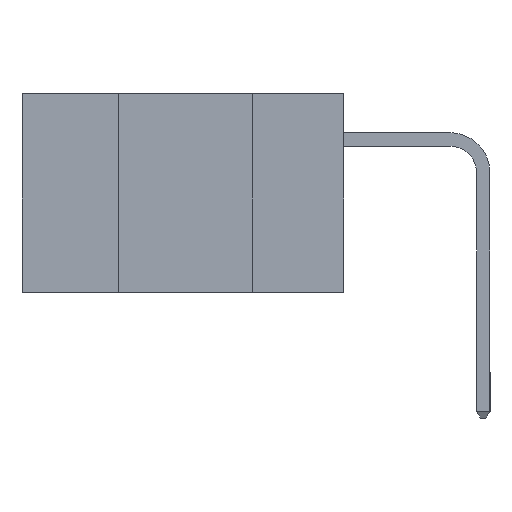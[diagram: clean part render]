
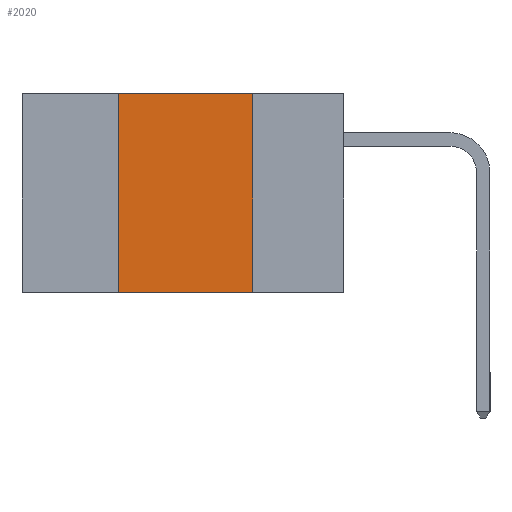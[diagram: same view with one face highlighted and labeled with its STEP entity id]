
A CAD part, left-side view. The second image highlights one B-rep face of the part: STEP entity #2020.
In plain terms, the highlighted planar face has unit normal (-1, 0, 0).
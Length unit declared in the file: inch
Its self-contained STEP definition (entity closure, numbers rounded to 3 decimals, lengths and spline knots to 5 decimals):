
#37 = CARTESIAN_POINT ( 'NONE',  ( 0., 0.6, 0. ) ) ;
#674 = EDGE_CURVE ( 'NONE', #14093, #16305, #2768, .T. ) ;
#2020 = ADVANCED_FACE ( 'NONE', ( #15001 ), #13443, .F. ) ;
#2191 = DIRECTION ( 'NONE',  ( 0., 0., 1. ) ) ;
#2768 = LINE ( 'NONE', #17792, #7282 ) ;
#3867 = ORIENTED_EDGE ( 'NONE', *, *, #10110, .F. ) ;
#4399 = ORIENTED_EDGE ( 'NONE', *, *, #674, .T. ) ;
#4702 = VECTOR ( 'NONE', #18523, 39.37008 ) ;
#6022 = EDGE_CURVE ( 'NONE', #7091, #16305, #18148, .T. ) ;
#6172 = DIRECTION ( 'NONE',  ( 1., 0., 0. ) ) ;
#6726 = CARTESIAN_POINT ( 'NONE',  ( 0., 0.17, -0.37 ) ) ;
#7091 = VERTEX_POINT ( 'NONE', #10139 ) ;
#7190 = LINE ( 'NONE', #17348, #14059 ) ;
#7282 = VECTOR ( 'NONE', #10734, 39.37008 ) ;
#7347 = CARTESIAN_POINT ( 'NONE',  ( 0., 0.17, -0.37 ) ) ;
#7876 = EDGE_CURVE ( 'NONE', #10659, #7091, #7190, .T. ) ;
#8228 = CARTESIAN_POINT ( 'NONE',  ( 0., 0.42, -0.37 ) ) ;
#8496 = ORIENTED_EDGE ( 'NONE', *, *, #7876, .F. ) ;
#8790 = CARTESIAN_POINT ( 'NONE',  ( 0., 0.42, 0. ) ) ;
#9874 = LINE ( 'NONE', #8228, #15904 ) ;
#10110 = EDGE_CURVE ( 'NONE', #14093, #10659, #9874, .T. ) ;
#10139 = CARTESIAN_POINT ( 'NONE',  ( 0., 0.17, 0. ) ) ;
#10659 = VERTEX_POINT ( 'NONE', #8790 ) ;
#10734 = DIRECTION ( 'NONE',  ( 0., -1., 0. ) ) ;
#11851 = CARTESIAN_POINT ( 'NONE',  ( 0., 0.42, -0.37 ) ) ;
#13099 = DIRECTION ( 'NONE',  ( 0., -1., 0. ) ) ;
#13404 = EDGE_LOOP ( 'NONE', ( #16418, #8496, #3867, #4399 ) ) ;
#13443 = PLANE ( 'NONE',  #16863 ) ;
#14059 = VECTOR ( 'NONE', #13099, 39.37008 ) ;
#14093 = VERTEX_POINT ( 'NONE', #11851 ) ;
#15001 = FACE_OUTER_BOUND ( 'NONE', #13404, .T. ) ;
#15904 = VECTOR ( 'NONE', #2191, 39.37008 ) ;
#16305 = VERTEX_POINT ( 'NONE', #7347 ) ;
#16418 = ORIENTED_EDGE ( 'NONE', *, *, #6022, .F. ) ;
#16863 = AXIS2_PLACEMENT_3D ( 'NONE', #37, #6172, #18071 ) ;
#17348 = CARTESIAN_POINT ( 'NONE',  ( 0., 0.6, 0. ) ) ;
#17792 = CARTESIAN_POINT ( 'NONE',  ( 0., 0.6, -0.37 ) ) ;
#18071 = DIRECTION ( 'NONE',  ( 0., 0., -1. ) ) ;
#18148 = LINE ( 'NONE', #6726, #4702 ) ;
#18523 = DIRECTION ( 'NONE',  ( 0., 0., -1. ) ) ;
